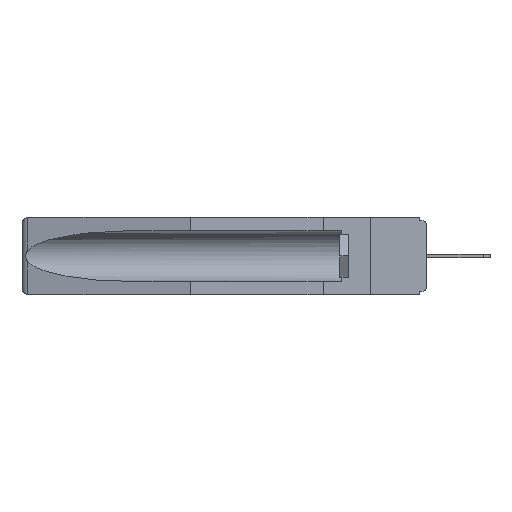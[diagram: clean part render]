
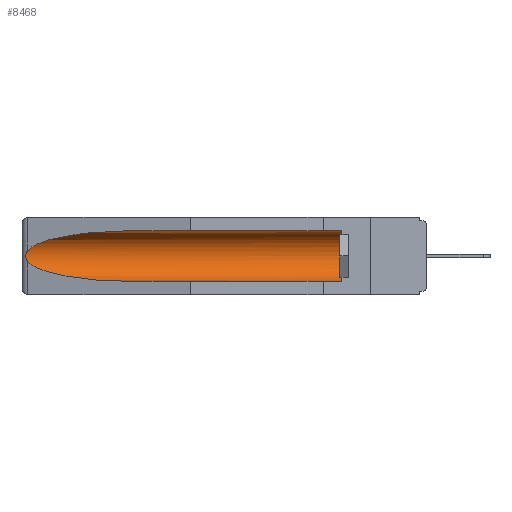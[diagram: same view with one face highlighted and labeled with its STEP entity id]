
A CAD part, left-side view. The second image highlights one B-rep face of the part: STEP entity #8468.
In plain terms, the highlighted cylindrical face has radius 2.857 mm (diameter 5.715 mm), a partial arc.
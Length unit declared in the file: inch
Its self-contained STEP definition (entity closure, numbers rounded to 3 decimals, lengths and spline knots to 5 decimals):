
#77 = CARTESIAN_POINT ( 'NONE',  ( 0.26537, 1.52718, -0.14972 ) ) ;
#154 = B_SPLINE_CURVE_WITH_KNOTS ( 'NONE', 3,
 ( #1603, #11613, #13087, #4436, #14506, #5890, #15916, #7358, #17328, #8785 ),
 .UNSPECIFIED., .F., .F.,
 ( 4, 2, 2, 2, 4 ),
 ( 0., 0.00029, 0.00058, 0.00087, 0.00117 ),
 .UNSPECIFIED. ) ;
#219 = FACE_OUTER_BOUND ( 'NONE', #4474, .T. ) ;
#502 = CARTESIAN_POINT ( 'NONE',  ( 0.155, 0.126, -0.284 ) ) ;
#1340 = CARTESIAN_POINT ( 'NONE',  ( 0.21114, 1.30732, -0.284 ) ) ;
#1423 = DIRECTION ( 'NONE',  ( 0., 1., 0. ) ) ;
#1603 = CARTESIAN_POINT ( 'NONE',  ( 0.26537, 1.52718, -0.14972 ) ) ;
#1764 = CARTESIAN_POINT ( 'NONE',  ( 0.21114, 1.30732, -0.059 ) ) ;
#2001 =( BOUNDED_CURVE ( )  B_SPLINE_CURVE ( 3, ( #4169, #14183, #1340, #5617 ),
 .UNSPECIFIED., .F., .T. ) 
 B_SPLINE_CURVE_WITH_KNOTS ( ( 4, 4 ),
 ( 0.1948, 1.5708 ),
 .UNSPECIFIED. ) 
 CURVE ( )  GEOMETRIC_REPRESENTATION_ITEM ( )  RATIONAL_B_SPLINE_CURVE ( ( 1., 0.848, 0.848, 1. ) ) 
 REPRESENTATION_ITEM ( '' )  );
#2108 = CARTESIAN_POINT ( 'NONE',  ( 0.155, -0.30754, -0.1715 ) ) ;
#2302 = VERTEX_POINT ( 'NONE', #13459 ) ;
#2361 =( BOUNDED_CURVE ( )  B_SPLINE_CURVE ( 3, ( #16062, #1764, #17485, #8947 ),
 .UNSPECIFIED., .F., .T. ) 
 B_SPLINE_CURVE_WITH_KNOTS ( ( 4, 4 ),
 ( 4.71239, 6.08839 ),
 .UNSPECIFIED. ) 
 CURVE ( )  GEOMETRIC_REPRESENTATION_ITEM ( )  RATIONAL_B_SPLINE_CURVE ( ( 1., 0.848, 0.848, 1. ) ) 
 REPRESENTATION_ITEM ( '' )  );
#2513 = VERTEX_POINT ( 'NONE', #77 ) ;
#3299 = ORIENTED_EDGE ( 'NONE', *, *, #12958, .T. ) ;
#4142 = CIRCLE ( 'NONE', #7131, 0.1125 ) ;
#4169 = CARTESIAN_POINT ( 'NONE',  ( 0.26537, 1.52718, -0.19328 ) ) ;
#4174 = CARTESIAN_POINT ( 'NONE',  ( 0.155, -0.30754, -0.284 ) ) ;
#4284 = EDGE_CURVE ( 'NONE', #6438, #2513, #2361, .T. ) ;
#4338 = CARTESIAN_POINT ( 'NONE',  ( 0.26537, 1.52718, -0.19328 ) ) ;
#4436 = CARTESIAN_POINT ( 'NONE',  ( 0.2673, 1.5327, -0.16383 ) ) ;
#4474 = EDGE_LOOP ( 'NONE', ( #4517, #3299, #17032, #7539, #14542, #12449 ) ) ;
#4517 = ORIENTED_EDGE ( 'NONE', *, *, #4284, .T. ) ;
#5474 = AXIS2_PLACEMENT_3D ( 'NONE', #2108, #6358, #9228 ) ;
#5617 = CARTESIAN_POINT ( 'NONE',  ( 0.155, 1.07973, -0.284 ) ) ;
#5775 = CARTESIAN_POINT ( 'NONE',  ( 0.155, 1.07973, -0.284 ) ) ;
#5890 = CARTESIAN_POINT ( 'NONE',  ( 0.2675, 1.53308, -0.17534 ) ) ;
#6358 = DIRECTION ( 'NONE',  ( 0., 1., 0. ) ) ;
#6438 = VERTEX_POINT ( 'NONE', #11131 ) ;
#6675 = DIRECTION ( 'NONE',  ( 0., -1., 0. ) ) ;
#6967 = EDGE_CURVE ( 'NONE', #7727, #15406, #2001, .T. ) ;
#7095 = DIRECTION ( 'NONE',  ( 0., 1., 0. ) ) ;
#7131 = AXIS2_PLACEMENT_3D ( 'NONE', #15262, #6675, #16659 ) ;
#7358 = CARTESIAN_POINT ( 'NONE',  ( 0.26655, 1.53094, -0.18657 ) ) ;
#7398 = CYLINDRICAL_SURFACE ( 'NONE', #5474, 0.1125 ) ;
#7539 = ORIENTED_EDGE ( 'NONE', *, *, #14711, .F. ) ;
#7727 = VERTEX_POINT ( 'NONE', #4338 ) ;
#8468 = ADVANCED_FACE ( 'NONE', ( #219 ), #7398, .F. ) ;
#8785 = CARTESIAN_POINT ( 'NONE',  ( 0.26537, 1.52718, -0.19328 ) ) ;
#8947 = CARTESIAN_POINT ( 'NONE',  ( 0.26537, 1.52718, -0.14972 ) ) ;
#9228 = DIRECTION ( 'NONE',  ( 0., 0., 1. ) ) ;
#9660 = LINE ( 'NONE', #4174, #13076 ) ;
#10477 = VERTEX_POINT ( 'NONE', #502 ) ;
#11131 = CARTESIAN_POINT ( 'NONE',  ( 0.155, 1.07973, -0.059 ) ) ;
#11613 = CARTESIAN_POINT ( 'NONE',  ( 0.26597, 1.52961, -0.15275 ) ) ;
#12449 = ORIENTED_EDGE ( 'NONE', *, *, #15361, .T. ) ;
#12958 = EDGE_CURVE ( 'NONE', #2513, #7727, #154, .T. ) ;
#13076 = VECTOR ( 'NONE', #7095, 39.37008 ) ;
#13087 = CARTESIAN_POINT ( 'NONE',  ( 0.26654, 1.53092, -0.15636 ) ) ;
#13278 = LINE ( 'NONE', #18502, #16558 ) ;
#13459 = CARTESIAN_POINT ( 'NONE',  ( 0.155, 0.126, -0.059 ) ) ;
#14183 = CARTESIAN_POINT ( 'NONE',  ( 0.25451, 1.48313, -0.24835 ) ) ;
#14506 = CARTESIAN_POINT ( 'NONE',  ( 0.2675, 1.53308, -0.16763 ) ) ;
#14542 = ORIENTED_EDGE ( 'NONE', *, *, #18376, .T. ) ;
#14711 = EDGE_CURVE ( 'NONE', #10477, #15406, #9660, .T. ) ;
#15262 = CARTESIAN_POINT ( 'NONE',  ( 0.155, 0.126, -0.1715 ) ) ;
#15361 = EDGE_CURVE ( 'NONE', #2302, #6438, #13278, .T. ) ;
#15406 = VERTEX_POINT ( 'NONE', #5775 ) ;
#15916 = CARTESIAN_POINT ( 'NONE',  ( 0.2673, 1.53269, -0.17917 ) ) ;
#16062 = CARTESIAN_POINT ( 'NONE',  ( 0.155, 1.07973, -0.059 ) ) ;
#16558 = VECTOR ( 'NONE', #1423, 39.37008 ) ;
#16659 = DIRECTION ( 'NONE',  ( 0., 0., 1. ) ) ;
#17032 = ORIENTED_EDGE ( 'NONE', *, *, #6967, .T. ) ;
#17328 = CARTESIAN_POINT ( 'NONE',  ( 0.26597, 1.5296, -0.19026 ) ) ;
#17485 = CARTESIAN_POINT ( 'NONE',  ( 0.25451, 1.48313, -0.09465 ) ) ;
#18376 = EDGE_CURVE ( 'NONE', #10477, #2302, #4142, .T. ) ;
#18502 = CARTESIAN_POINT ( 'NONE',  ( 0.155, -0.30754, -0.059 ) ) ;
